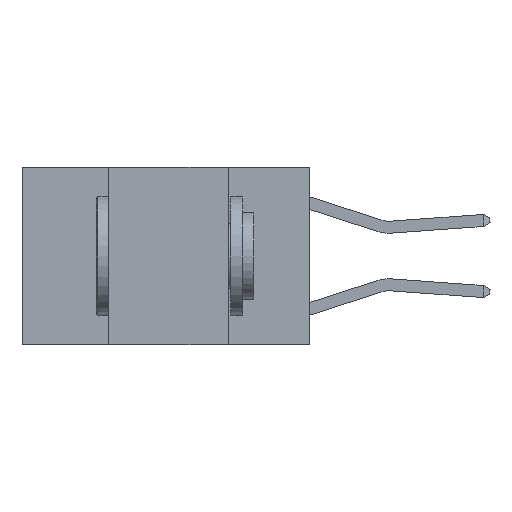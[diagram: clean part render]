
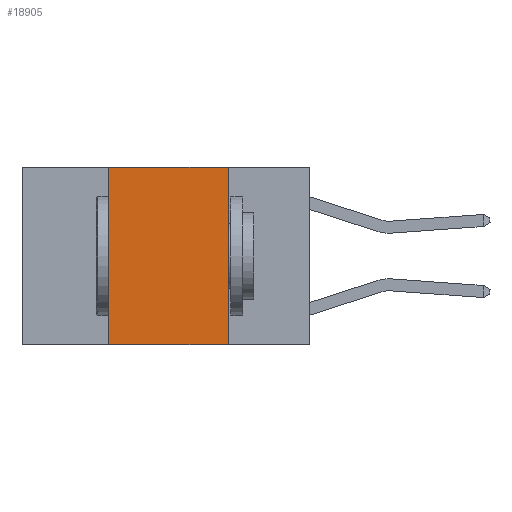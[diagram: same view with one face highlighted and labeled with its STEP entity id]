
A CAD part, left-side view. The second image highlights one B-rep face of the part: STEP entity #18905.
In plain terms, the highlighted planar face has unit normal (-1, 0, 0).
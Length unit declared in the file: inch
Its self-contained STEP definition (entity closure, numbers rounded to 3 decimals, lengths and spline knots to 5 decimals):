
#804 = ORIENTED_EDGE ( 'NONE', *, *, #3193, .F. ) ;
#886 = ORIENTED_EDGE ( 'NONE', *, *, #9900, .F. ) ;
#1935 = DIRECTION ( 'NONE',  ( 1., 0., 0. ) ) ;
#2779 = LINE ( 'NONE', #27661, #23502 ) ;
#2921 = VECTOR ( 'NONE', #18402, 39.37008 ) ;
#3193 = EDGE_CURVE ( 'NONE', #7802, #19374, #2779, .T. ) ;
#6691 = VECTOR ( 'NONE', #16329, 39.37008 ) ;
#6807 = LINE ( 'NONE', #26904, #2921 ) ;
#7802 = VERTEX_POINT ( 'NONE', #23537 ) ;
#8737 = CARTESIAN_POINT ( 'NONE',  ( 0., 0.6, 0. ) ) ;
#9445 = DIRECTION ( 'NONE',  ( 0., 0., -1. ) ) ;
#9900 = EDGE_CURVE ( 'NONE', #25827, #7802, #6807, .T. ) ;
#10568 = CARTESIAN_POINT ( 'NONE',  ( 0., 0.42, -0.37 ) ) ;
#10733 = LINE ( 'NONE', #27168, #11037 ) ;
#11037 = VECTOR ( 'NONE', #15741, 39.37008 ) ;
#11426 = DIRECTION ( 'NONE',  ( 0., 0., -1. ) ) ;
#12477 = CARTESIAN_POINT ( 'NONE',  ( 0., 0.42, 0. ) ) ;
#13264 = VERTEX_POINT ( 'NONE', #10568 ) ;
#14054 = LINE ( 'NONE', #27316, #6691 ) ;
#15741 = DIRECTION ( 'NONE',  ( 0., -1., 0. ) ) ;
#15989 = FACE_OUTER_BOUND ( 'NONE', #26966, .T. ) ;
#16329 = DIRECTION ( 'NONE',  ( 0., 0., 1. ) ) ;
#18121 = ORIENTED_EDGE ( 'NONE', *, *, #21660, .T. ) ;
#18283 = ORIENTED_EDGE ( 'NONE', *, *, #22022, .F. ) ;
#18402 = DIRECTION ( 'NONE',  ( 0., -1., 0. ) ) ;
#18905 = ADVANCED_FACE ( 'NONE', ( #15989 ), #25131, .F. ) ;
#19374 = VERTEX_POINT ( 'NONE', #29636 ) ;
#20555 = AXIS2_PLACEMENT_3D ( 'NONE', #8737, #1935, #11426 ) ;
#21660 = EDGE_CURVE ( 'NONE', #13264, #19374, #10733, .T. ) ;
#22022 = EDGE_CURVE ( 'NONE', #13264, #25827, #14054, .T. ) ;
#23502 = VECTOR ( 'NONE', #9445, 39.37008 ) ;
#23537 = CARTESIAN_POINT ( 'NONE',  ( 0., 0.17, 0. ) ) ;
#25131 = PLANE ( 'NONE',  #20555 ) ;
#25827 = VERTEX_POINT ( 'NONE', #12477 ) ;
#26904 = CARTESIAN_POINT ( 'NONE',  ( 0., 0.6, 0. ) ) ;
#26966 = EDGE_LOOP ( 'NONE', ( #804, #886, #18283, #18121 ) ) ;
#27168 = CARTESIAN_POINT ( 'NONE',  ( 0., 0.6, -0.37 ) ) ;
#27316 = CARTESIAN_POINT ( 'NONE',  ( 0., 0.42, 0. ) ) ;
#27661 = CARTESIAN_POINT ( 'NONE',  ( 0., 0.17, 0. ) ) ;
#29636 = CARTESIAN_POINT ( 'NONE',  ( 0., 0.17, -0.37 ) ) ;
